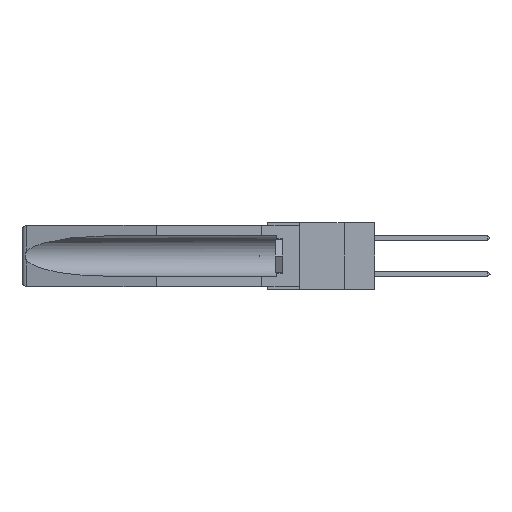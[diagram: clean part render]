
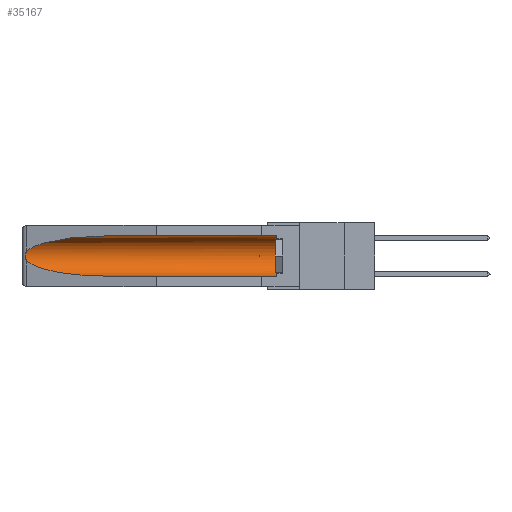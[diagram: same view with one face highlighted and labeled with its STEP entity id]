
A CAD part, left-side view. The second image highlights one B-rep face of the part: STEP entity #35167.
In plain terms, the highlighted cylindrical face has radius 2.857 mm (diameter 5.715 mm), a partial arc.
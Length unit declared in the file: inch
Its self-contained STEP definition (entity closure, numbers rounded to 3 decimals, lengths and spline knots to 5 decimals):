
#780 = CARTESIAN_POINT ( 'NONE',  ( 0.26537, 1.52718, -0.14972 ) ) ;
#1785 = EDGE_LOOP ( 'NONE', ( #25527, #17508, #8552, #22840, #9260, #35187 ) ) ;
#2640 = CARTESIAN_POINT ( 'NONE',  ( 0.26537, 1.52718, -0.14972 ) ) ;
#2976 = CARTESIAN_POINT ( 'NONE',  ( 0.155, 1.07973, -0.284 ) ) ;
#3829 = CARTESIAN_POINT ( 'NONE',  ( 0.155, 1.07973, -0.284 ) ) ;
#4413 =( BOUNDED_CURVE ( )  B_SPLINE_CURVE ( 3, ( #25323, #32714, #11511, #2640 ),
 .UNSPECIFIED., .F., .T. ) 
 B_SPLINE_CURVE_WITH_KNOTS ( ( 4, 4 ),
 ( 4.71239, 6.08839 ),
 .UNSPECIFIED. ) 
 CURVE ( )  GEOMETRIC_REPRESENTATION_ITEM ( )  RATIONAL_B_SPLINE_CURVE ( ( 1., 0.848, 0.848, 1. ) ) 
 REPRESENTATION_ITEM ( '' )  );
#5139 = EDGE_CURVE ( 'NONE', #27403, #11790, #6925, .T. ) ;
#5977 = CARTESIAN_POINT ( 'NONE',  ( 0.26597, 1.5296, -0.19026 ) ) ;
#6322 = CARTESIAN_POINT ( 'NONE',  ( 0.155, -0.30754, -0.284 ) ) ;
#6925 = LINE ( 'NONE', #6322, #12000 ) ;
#8415 = DIRECTION ( 'NONE',  ( 0., -1., 0. ) ) ;
#8552 = ORIENTED_EDGE ( 'NONE', *, *, #18516, .T. ) ;
#9038 = DIRECTION ( 'NONE',  ( 0., 1., 0. ) ) ;
#9129 = CARTESIAN_POINT ( 'NONE',  ( 0.2673, 1.53269, -0.17917 ) ) ;
#9260 = ORIENTED_EDGE ( 'NONE', *, *, #27654, .T. ) ;
#10073 = AXIS2_PLACEMENT_3D ( 'NONE', #19215, #8415, #11263 ) ;
#10081 = EDGE_CURVE ( 'NONE', #21959, #26791, #4413, .T. ) ;
#11263 = DIRECTION ( 'NONE',  ( 0., 0., 1. ) ) ;
#11314 = CYLINDRICAL_SURFACE ( 'NONE', #20454, 0.1125 ) ;
#11511 = CARTESIAN_POINT ( 'NONE',  ( 0.25451, 1.48313, -0.09465 ) ) ;
#11532 = CARTESIAN_POINT ( 'NONE',  ( 0.26654, 1.53092, -0.15636 ) ) ;
#11637 = CARTESIAN_POINT ( 'NONE',  ( 0.155, 1.07973, -0.059 ) ) ;
#11646 = CARTESIAN_POINT ( 'NONE',  ( 0.26655, 1.53094, -0.18657 ) ) ;
#11790 = VERTEX_POINT ( 'NONE', #3829 ) ;
#12000 = VECTOR ( 'NONE', #9038, 39.37008 ) ;
#13735 = DIRECTION ( 'NONE',  ( 0., 0., 1. ) ) ;
#14136 = CARTESIAN_POINT ( 'NONE',  ( 0.155, 0.126, -0.059 ) ) ;
#14143 = CARTESIAN_POINT ( 'NONE',  ( 0.26537, 1.52718, -0.19328 ) ) ;
#17077 = CARTESIAN_POINT ( 'NONE',  ( 0.2675, 1.53308, -0.16763 ) ) ;
#17508 = ORIENTED_EDGE ( 'NONE', *, *, #33849, .T. ) ;
#17917 = VERTEX_POINT ( 'NONE', #14136 ) ;
#18494 = LINE ( 'NONE', #25081, #22360 ) ;
#18516 = EDGE_CURVE ( 'NONE', #21406, #11790, #20736, .T. ) ;
#19215 = CARTESIAN_POINT ( 'NONE',  ( 0.155, 0.126, -0.1715 ) ) ;
#19843 = CARTESIAN_POINT ( 'NONE',  ( 0.2673, 1.5327, -0.16383 ) ) ;
#20234 = FACE_OUTER_BOUND ( 'NONE', #1785, .T. ) ;
#20454 = AXIS2_PLACEMENT_3D ( 'NONE', #24592, #24824, #13735 ) ;
#20736 =( BOUNDED_CURVE ( )  B_SPLINE_CURVE ( 3, ( #32580, #30050, #32810, #2976 ),
 .UNSPECIFIED., .F., .F. ) 
 B_SPLINE_CURVE_WITH_KNOTS ( ( 4, 4 ),
 ( 0.1948, 1.5708 ),
 .UNSPECIFIED. ) 
 CURVE ( )  GEOMETRIC_REPRESENTATION_ITEM ( )  RATIONAL_B_SPLINE_CURVE ( ( 1., 0.848, 0.848, 1. ) ) 
 REPRESENTATION_ITEM ( '' )  );
#21406 = VERTEX_POINT ( 'NONE', #22026 ) ;
#21959 = VERTEX_POINT ( 'NONE', #11637 ) ;
#22026 = CARTESIAN_POINT ( 'NONE',  ( 0.26537, 1.52718, -0.19328 ) ) ;
#22360 = VECTOR ( 'NONE', #25426, 39.37008 ) ;
#22840 = ORIENTED_EDGE ( 'NONE', *, *, #5139, .F. ) ;
#23203 = CARTESIAN_POINT ( 'NONE',  ( 0.26537, 1.52718, -0.14972 ) ) ;
#24592 = CARTESIAN_POINT ( 'NONE',  ( 0.155, -0.30754, -0.1715 ) ) ;
#24824 = DIRECTION ( 'NONE',  ( 0., 1., 0. ) ) ;
#25081 = CARTESIAN_POINT ( 'NONE',  ( 0.155, -0.30754, -0.059 ) ) ;
#25229 = CARTESIAN_POINT ( 'NONE',  ( 0.2675, 1.53308, -0.17534 ) ) ;
#25323 = CARTESIAN_POINT ( 'NONE',  ( 0.155, 1.07973, -0.059 ) ) ;
#25426 = DIRECTION ( 'NONE',  ( 0., 1., 0. ) ) ;
#25527 = ORIENTED_EDGE ( 'NONE', *, *, #10081, .T. ) ;
#26508 = CIRCLE ( 'NONE', #10073, 0.1125 ) ;
#26791 = VERTEX_POINT ( 'NONE', #23203 ) ;
#27403 = VERTEX_POINT ( 'NONE', #31871 ) ;
#27654 = EDGE_CURVE ( 'NONE', #27403, #17917, #26508, .T. ) ;
#27743 = CARTESIAN_POINT ( 'NONE',  ( 0.26597, 1.52961, -0.15275 ) ) ;
#30050 = CARTESIAN_POINT ( 'NONE',  ( 0.25451, 1.48313, -0.24835 ) ) ;
#31871 = CARTESIAN_POINT ( 'NONE',  ( 0.155, 0.126, -0.284 ) ) ;
#32580 = CARTESIAN_POINT ( 'NONE',  ( 0.26537, 1.52718, -0.19328 ) ) ;
#32714 = CARTESIAN_POINT ( 'NONE',  ( 0.21114, 1.30732, -0.059 ) ) ;
#32810 = CARTESIAN_POINT ( 'NONE',  ( 0.21114, 1.30732, -0.284 ) ) ;
#33849 = EDGE_CURVE ( 'NONE', #26791, #21406, #34689, .T. ) ;
#34398 = EDGE_CURVE ( 'NONE', #17917, #21959, #18494, .T. ) ;
#34689 = B_SPLINE_CURVE_WITH_KNOTS ( 'NONE', 3,
 ( #780, #27743, #11532, #19843, #17077, #25229, #9129, #11646, #5977, #14143 ),
 .UNSPECIFIED., .F., .F.,
 ( 4, 2, 2, 2, 4 ),
 ( 0., 0.00029, 0.00058, 0.00087, 0.00117 ),
 .UNSPECIFIED. ) ;
#35167 = ADVANCED_FACE ( 'NONE', ( #20234 ), #11314, .F. ) ;
#35187 = ORIENTED_EDGE ( 'NONE', *, *, #34398, .T. ) ;
